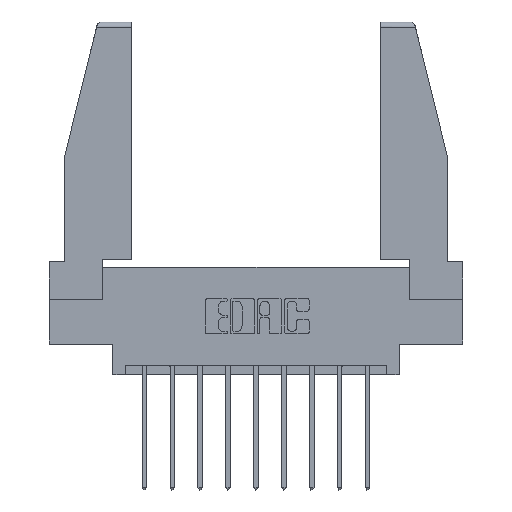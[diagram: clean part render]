
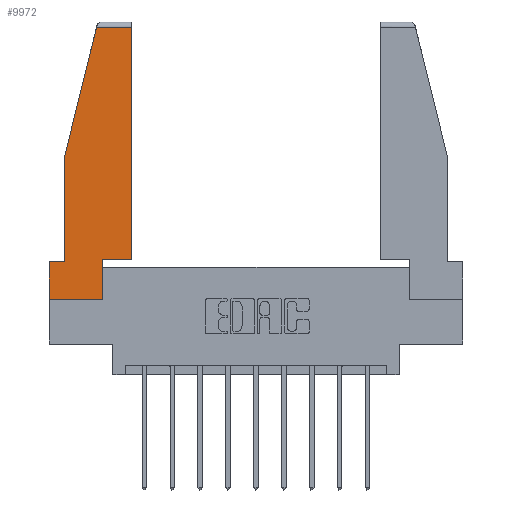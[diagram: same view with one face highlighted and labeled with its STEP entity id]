
A CAD part, top view. The second image highlights one B-rep face of the part: STEP entity #9972.
In plain terms, the highlighted planar face has unit normal (0, 0, 1).
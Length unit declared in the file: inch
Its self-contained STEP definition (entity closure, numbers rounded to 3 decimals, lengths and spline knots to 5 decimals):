
#122 = CARTESIAN_POINT ( 'NONE',  ( 0., 0.21, 0. ) ) ;
#375 = LINE ( 'NONE', #917, #5031 ) ;
#439 = CARTESIAN_POINT ( 'NONE',  ( 0.086, 0.8, 0. ) ) ;
#661 = ORIENTED_EDGE ( 'NONE', *, *, #845, .T. ) ;
#838 = DIRECTION ( 'NONE',  ( 0., 1., 0. ) ) ;
#845 = EDGE_CURVE ( 'NONE', #4990, #9915, #13173, .T. ) ;
#917 = CARTESIAN_POINT ( 'NONE',  ( 0.271, 1.55, 0. ) ) ;
#1167 = VERTEX_POINT ( 'NONE', #9188 ) ;
#1174 = DIRECTION ( 'NONE',  ( 1., 0., 0. ) ) ;
#1197 = CARTESIAN_POINT ( 'NONE',  ( 0., 0.21, 0. ) ) ;
#1212 = CARTESIAN_POINT ( 'NONE',  ( 0.2636, 1.52, 0. ) ) ;
#1244 = EDGE_CURVE ( 'NONE', #2208, #2854, #2803, .T. ) ;
#1361 = ORIENTED_EDGE ( 'NONE', *, *, #1765, .T. ) ;
#1382 = EDGE_CURVE ( 'NONE', #7358, #10523, #12826, .T. ) ;
#1706 = CARTESIAN_POINT ( 'NONE',  ( 0., 0.21, 0. ) ) ;
#1765 = EDGE_CURVE ( 'NONE', #8169, #4990, #1964, .T. ) ;
#1964 = LINE ( 'NONE', #6162, #9301 ) ;
#2167 = VERTEX_POINT ( 'NONE', #439 ) ;
#2208 = VERTEX_POINT ( 'NONE', #13247 ) ;
#2565 = LINE ( 'NONE', #1197, #7073 ) ;
#2604 = VECTOR ( 'NONE', #1174, 39.37008 ) ;
#2678 = DIRECTION ( 'NONE',  ( 0., -1., 0. ) ) ;
#2803 = LINE ( 'NONE', #9635, #13333 ) ;
#2854 = VERTEX_POINT ( 'NONE', #4098 ) ;
#3183 = ORIENTED_EDGE ( 'NONE', *, *, #8766, .T. ) ;
#3263 = CARTESIAN_POINT ( 'NONE',  ( 0., 0., 0. ) ) ;
#3901 = CARTESIAN_POINT ( 'NONE',  ( 0., 0., 0. ) ) ;
#4098 = CARTESIAN_POINT ( 'NONE',  ( 0.297, 0.223, 0. ) ) ;
#4188 = EDGE_CURVE ( 'NONE', #2854, #8169, #11916, .T. ) ;
#4208 = AXIS2_PLACEMENT_3D ( 'NONE', #5832, #8122, #11153 ) ;
#4261 = ORIENTED_EDGE ( 'NONE', *, *, #1244, .T. ) ;
#4544 = VECTOR ( 'NONE', #13437, 39.37008 ) ;
#4787 = DIRECTION ( 'NONE',  ( -1., 0., 0. ) ) ;
#4990 = VERTEX_POINT ( 'NONE', #9125 ) ;
#5031 = VECTOR ( 'NONE', #12694, 39.37008 ) ;
#5832 = CARTESIAN_POINT ( 'NONE',  ( 0., 0., 0. ) ) ;
#6162 = CARTESIAN_POINT ( 'NONE',  ( 0.461, 0.223, 0. ) ) ;
#6315 = ORIENTED_EDGE ( 'NONE', *, *, #4188, .T. ) ;
#6583 = DIRECTION ( 'NONE',  ( 0., -1., 0. ) ) ;
#6593 = ORIENTED_EDGE ( 'NONE', *, *, #7926, .T. ) ;
#6668 = VECTOR ( 'NONE', #4787, 39.37008 ) ;
#7073 = VECTOR ( 'NONE', #12963, 39.37008 ) ;
#7358 = VERTEX_POINT ( 'NONE', #1706 ) ;
#7641 = EDGE_CURVE ( 'NONE', #1167, #7358, #2565, .T. ) ;
#7926 = EDGE_CURVE ( 'NONE', #2167, #1167, #10896, .T. ) ;
#8029 = EDGE_LOOP ( 'NONE', ( #1361, #661, #3183, #6593, #11328, #10633, #11130, #4261, #6315 ) ) ;
#8122 = DIRECTION ( 'NONE',  ( 0., 0., 1. ) ) ;
#8169 = VERTEX_POINT ( 'NONE', #12847 ) ;
#8766 = EDGE_CURVE ( 'NONE', #9915, #2167, #375, .T. ) ;
#9125 = CARTESIAN_POINT ( 'NONE',  ( 0.461, 1.52, 0. ) ) ;
#9141 = VECTOR ( 'NONE', #6583, 39.37008 ) ;
#9188 = CARTESIAN_POINT ( 'NONE',  ( 0.086, 0.21, 0. ) ) ;
#9301 = VECTOR ( 'NONE', #838, 39.37008 ) ;
#9635 = CARTESIAN_POINT ( 'NONE',  ( 0.297, 0., 0. ) ) ;
#9915 = VERTEX_POINT ( 'NONE', #1212 ) ;
#9972 = ADVANCED_FACE ( 'NONE', ( #13196 ), #10210, .T. ) ;
#10091 = CARTESIAN_POINT ( 'NONE',  ( 0.086, 0.8, 0. ) ) ;
#10197 = CARTESIAN_POINT ( 'NONE',  ( 0.297, 0.223, 0. ) ) ;
#10210 = PLANE ( 'NONE',  #4208 ) ;
#10523 = VERTEX_POINT ( 'NONE', #3901 ) ;
#10557 = VECTOR ( 'NONE', #2678, 39.37008 ) ;
#10633 = ORIENTED_EDGE ( 'NONE', *, *, #1382, .T. ) ;
#10896 = LINE ( 'NONE', #10091, #10557 ) ;
#11130 = ORIENTED_EDGE ( 'NONE', *, *, #12229, .T. ) ;
#11152 = CARTESIAN_POINT ( 'NONE',  ( 0., 1.52, 0. ) ) ;
#11153 = DIRECTION ( 'NONE',  ( 1., 0., 0. ) ) ;
#11273 = LINE ( 'NONE', #3263, #2604 ) ;
#11328 = ORIENTED_EDGE ( 'NONE', *, *, #7641, .T. ) ;
#11790 = DIRECTION ( 'NONE',  ( 0., 1., 0. ) ) ;
#11916 = LINE ( 'NONE', #10197, #4544 ) ;
#12229 = EDGE_CURVE ( 'NONE', #10523, #2208, #11273, .T. ) ;
#12694 = DIRECTION ( 'NONE',  ( -0.239, -0.971, 0. ) ) ;
#12826 = LINE ( 'NONE', #122, #9141 ) ;
#12847 = CARTESIAN_POINT ( 'NONE',  ( 0.461, 0.223, 0. ) ) ;
#12963 = DIRECTION ( 'NONE',  ( -1., 0., 0. ) ) ;
#13173 = LINE ( 'NONE', #11152, #6668 ) ;
#13196 = FACE_OUTER_BOUND ( 'NONE', #8029, .T. ) ;
#13247 = CARTESIAN_POINT ( 'NONE',  ( 0.297, 0., 0. ) ) ;
#13333 = VECTOR ( 'NONE', #11790, 39.37008 ) ;
#13437 = DIRECTION ( 'NONE',  ( 1., 0., 0. ) ) ;
